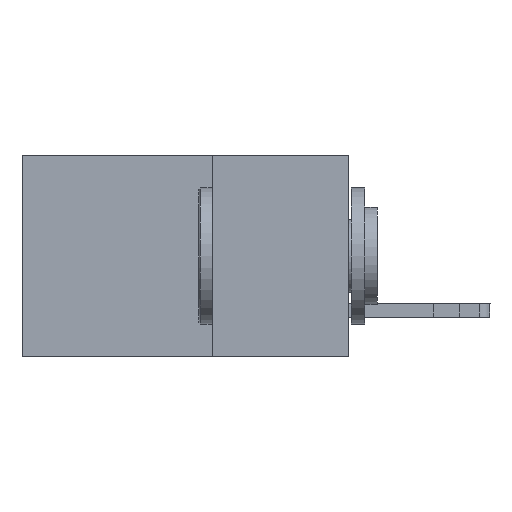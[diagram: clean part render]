
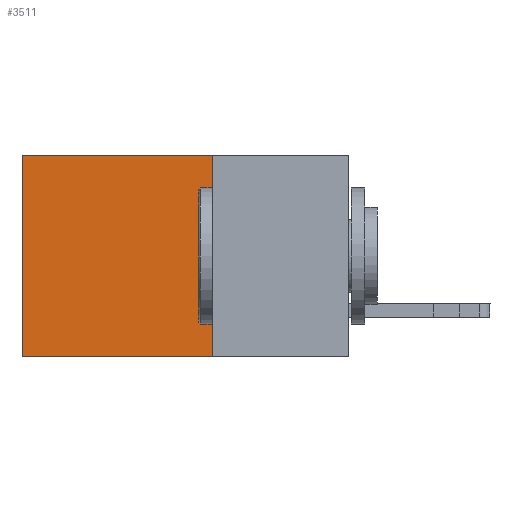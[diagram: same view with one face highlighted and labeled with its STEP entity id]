
A CAD part, left-side view. The second image highlights one B-rep face of the part: STEP entity #3511.
In plain terms, the highlighted planar face has unit normal (-1, 0, 0).
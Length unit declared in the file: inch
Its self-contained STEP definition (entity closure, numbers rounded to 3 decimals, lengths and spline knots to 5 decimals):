
#231 = CARTESIAN_POINT ( 'NONE',  ( 0.2615, 0.25, -0.37 ) ) ;
#1629 = LINE ( 'NONE', #6161, #3772 ) ;
#1935 = VERTEX_POINT ( 'NONE', #2100 ) ;
#2100 = CARTESIAN_POINT ( 'NONE',  ( 0.2615, 0.25, -0.37 ) ) ;
#2520 = DIRECTION ( 'NONE',  ( 0., 1., 0. ) ) ;
#2913 = VERTEX_POINT ( 'NONE', #8135 ) ;
#3416 = DIRECTION ( 'NONE',  ( 0., 0., -1. ) ) ;
#3511 = ADVANCED_FACE ( 'NONE', ( #5761 ), #4744, .F. ) ;
#3631 = ORIENTED_EDGE ( 'NONE', *, *, #5785, .F. ) ;
#3683 = DIRECTION ( 'NONE',  ( 0., 0., -1. ) ) ;
#3772 = VECTOR ( 'NONE', #3416, 39.37008 ) ;
#4042 = EDGE_CURVE ( 'NONE', #4529, #1935, #1629, .T. ) ;
#4206 = CARTESIAN_POINT ( 'NONE',  ( 0.2615, 0.6, 0. ) ) ;
#4338 = AXIS2_PLACEMENT_3D ( 'NONE', #231, #9420, #3683 ) ;
#4529 = VERTEX_POINT ( 'NONE', #7886 ) ;
#4744 = PLANE ( 'NONE',  #4338 ) ;
#5213 = VERTEX_POINT ( 'NONE', #4206 ) ;
#5630 = EDGE_CURVE ( 'NONE', #4529, #5213, #7709, .T. ) ;
#5761 = FACE_OUTER_BOUND ( 'NONE', #11336, .T. ) ;
#5785 = EDGE_CURVE ( 'NONE', #1935, #2913, #6208, .T. ) ;
#6086 = VECTOR ( 'NONE', #2520, 39.37008 ) ;
#6161 = CARTESIAN_POINT ( 'NONE',  ( 0.2615, 0.25, -0.37 ) ) ;
#6208 = LINE ( 'NONE', #8787, #6086 ) ;
#6237 = CARTESIAN_POINT ( 'NONE',  ( 0.2615, 0.6, -0.37 ) ) ;
#6319 = ORIENTED_EDGE ( 'NONE', *, *, #4042, .F. ) ;
#6807 = CARTESIAN_POINT ( 'NONE',  ( 0.2615, 0.25, 0. ) ) ;
#6958 = DIRECTION ( 'NONE',  ( 0., 0., -1. ) ) ;
#7433 = ORIENTED_EDGE ( 'NONE', *, *, #5630, .T. ) ;
#7709 = LINE ( 'NONE', #6807, #10289 ) ;
#7886 = CARTESIAN_POINT ( 'NONE',  ( 0.2615, 0.25, 0. ) ) ;
#8135 = CARTESIAN_POINT ( 'NONE',  ( 0.2615, 0.6, -0.37 ) ) ;
#8533 = ORIENTED_EDGE ( 'NONE', *, *, #10207, .T. ) ;
#8787 = CARTESIAN_POINT ( 'NONE',  ( 0.2615, 0.25, -0.37 ) ) ;
#9397 = DIRECTION ( 'NONE',  ( 0., 1., 0. ) ) ;
#9420 = DIRECTION ( 'NONE',  ( 1., 0., 0. ) ) ;
#9959 = VECTOR ( 'NONE', #6958, 39.37008 ) ;
#10207 = EDGE_CURVE ( 'NONE', #5213, #2913, #10615, .T. ) ;
#10289 = VECTOR ( 'NONE', #9397, 39.37008 ) ;
#10615 = LINE ( 'NONE', #6237, #9959 ) ;
#11336 = EDGE_LOOP ( 'NONE', ( #8533, #3631, #6319, #7433 ) ) ;
